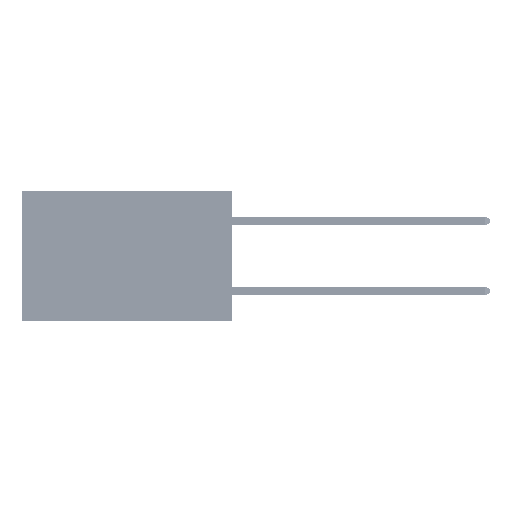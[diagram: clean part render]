
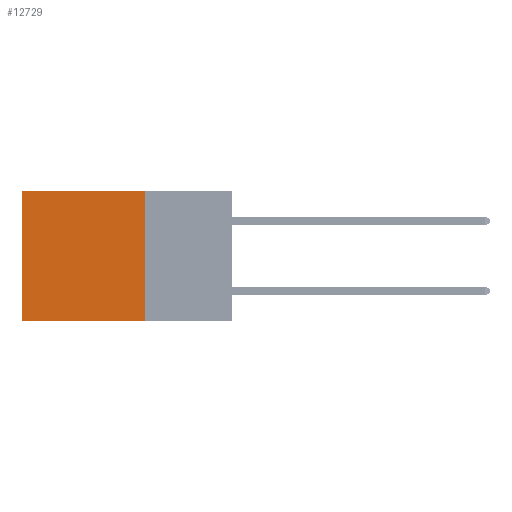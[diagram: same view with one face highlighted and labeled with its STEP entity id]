
A CAD part, left-side view. The second image highlights one B-rep face of the part: STEP entity #12729.
In plain terms, the highlighted planar face has unit normal (-1, 0, 0).
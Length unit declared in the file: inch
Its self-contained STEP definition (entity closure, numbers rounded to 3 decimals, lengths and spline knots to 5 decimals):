
#284 = EDGE_CURVE ( 'NONE', #39788, #41420, #30960, .T. ) ;
#1256 = CARTESIAN_POINT ( 'NONE',  ( 0.2875, 0.25, -0.37 ) ) ;
#3947 = ORIENTED_EDGE ( 'NONE', *, *, #35774, .F. ) ;
#9788 = DIRECTION ( 'NONE',  ( 1., 0., 0. ) ) ;
#10074 = DIRECTION ( 'NONE',  ( 0., 1., 0. ) ) ;
#11174 = DIRECTION ( 'NONE',  ( 0., 0., -1. ) ) ;
#11700 = ORIENTED_EDGE ( 'NONE', *, *, #284, .T. ) ;
#12729 = ADVANCED_FACE ( 'NONE', ( #17430 ), #13742, .F. ) ;
#13742 = PLANE ( 'NONE',  #34528 ) ;
#15527 = VECTOR ( 'NONE', #40972, 39.37008 ) ;
#17023 = VERTEX_POINT ( 'NONE', #24191 ) ;
#17430 = FACE_OUTER_BOUND ( 'NONE', #40262, .T. ) ;
#18221 = VECTOR ( 'NONE', #11174, 39.37008 ) ;
#18408 = CARTESIAN_POINT ( 'NONE',  ( 0.2875, 0.6, 0. ) ) ;
#20418 = LINE ( 'NONE', #32554, #15527 ) ;
#21194 = DIRECTION ( 'NONE',  ( 0., 1., 0. ) ) ;
#23112 = VECTOR ( 'NONE', #21194, 39.37008 ) ;
#24191 = CARTESIAN_POINT ( 'NONE',  ( 0.2875, 0.25, 0. ) ) ;
#25170 = LINE ( 'NONE', #41239, #23112 ) ;
#25880 = DIRECTION ( 'NONE',  ( 0., 0., -1. ) ) ;
#26985 = VECTOR ( 'NONE', #10074, 39.37008 ) ;
#30960 = LINE ( 'NONE', #31233, #18221 ) ;
#31233 = CARTESIAN_POINT ( 'NONE',  ( 0.2875, 0.6, 0. ) ) ;
#32554 = CARTESIAN_POINT ( 'NONE',  ( 0.2875, 0.25, 0. ) ) ;
#33701 = VERTEX_POINT ( 'NONE', #1256 ) ;
#33791 = CARTESIAN_POINT ( 'NONE',  ( 0.2875, 0.25, 0. ) ) ;
#34528 = AXIS2_PLACEMENT_3D ( 'NONE', #33791, #9788, #25880 ) ;
#35774 = EDGE_CURVE ( 'NONE', #17023, #33701, #20418, .T. ) ;
#35951 = EDGE_CURVE ( 'NONE', #33701, #41420, #25170, .T. ) ;
#38280 = CARTESIAN_POINT ( 'NONE',  ( 0.2875, 0.25, 0. ) ) ;
#39788 = VERTEX_POINT ( 'NONE', #18408 ) ;
#40262 = EDGE_LOOP ( 'NONE', ( #11700, #44894, #3947, #50340 ) ) ;
#40972 = DIRECTION ( 'NONE',  ( 0., 0., -1. ) ) ;
#41239 = CARTESIAN_POINT ( 'NONE',  ( 0.2875, 0.25, -0.37 ) ) ;
#41420 = VERTEX_POINT ( 'NONE', #47797 ) ;
#44894 = ORIENTED_EDGE ( 'NONE', *, *, #35951, .F. ) ;
#46241 = EDGE_CURVE ( 'NONE', #17023, #39788, #49345, .T. ) ;
#47797 = CARTESIAN_POINT ( 'NONE',  ( 0.2875, 0.6, -0.37 ) ) ;
#49345 = LINE ( 'NONE', #38280, #26985 ) ;
#50340 = ORIENTED_EDGE ( 'NONE', *, *, #46241, .T. ) ;
